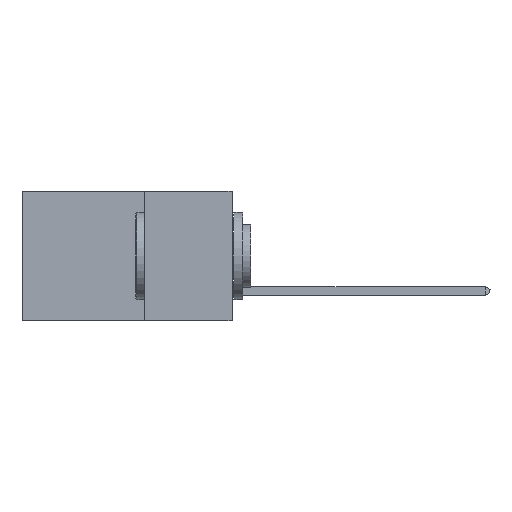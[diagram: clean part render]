
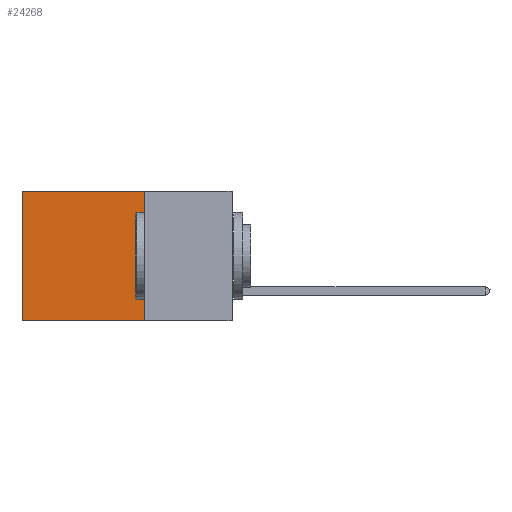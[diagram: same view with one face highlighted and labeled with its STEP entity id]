
A CAD part, left-side view. The second image highlights one B-rep face of the part: STEP entity #24268.
In plain terms, the highlighted planar face has unit normal (-1, 0, 0).
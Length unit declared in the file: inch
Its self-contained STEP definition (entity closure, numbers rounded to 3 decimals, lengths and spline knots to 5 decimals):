
#7 = ORIENTED_EDGE ( 'NONE', *, *, #32468, .F. ) ;
#104 = LINE ( 'NONE', #16611, #7151 ) ;
#862 = VERTEX_POINT ( 'NONE', #12996 ) ;
#2606 = LINE ( 'NONE', #25708, #44000 ) ;
#4894 = EDGE_CURVE ( 'NONE', #24245, #862, #31543, .T. ) ;
#5495 = CARTESIAN_POINT ( 'NONE',  ( 0.2875, 0.25, 0. ) ) ;
#5816 = CARTESIAN_POINT ( 'NONE',  ( 0.2875, 0.25, 0. ) ) ;
#6486 = VECTOR ( 'NONE', #27699, 39.37008 ) ;
#6869 = ORIENTED_EDGE ( 'NONE', *, *, #26207, .T. ) ;
#7151 = VECTOR ( 'NONE', #40931, 39.37008 ) ;
#7490 = CARTESIAN_POINT ( 'NONE',  ( 0.2875, 0.25, -0.37 ) ) ;
#8475 = DIRECTION ( 'NONE',  ( 0., 0., -1. ) ) ;
#10782 = VECTOR ( 'NONE', #38399, 39.37008 ) ;
#11409 = VERTEX_POINT ( 'NONE', #7490 ) ;
#12547 = DIRECTION ( 'NONE',  ( 0., 0., -1. ) ) ;
#12996 = CARTESIAN_POINT ( 'NONE',  ( 0.2875, 0.6, 0. ) ) ;
#16611 = CARTESIAN_POINT ( 'NONE',  ( 0.2875, 0.25, -0.37 ) ) ;
#19975 = EDGE_LOOP ( 'NONE', ( #6869, #7, #23377, #36770 ) ) ;
#21014 = EDGE_CURVE ( 'NONE', #24245, #11409, #2606, .T. ) ;
#23377 = ORIENTED_EDGE ( 'NONE', *, *, #21014, .F. ) ;
#24245 = VERTEX_POINT ( 'NONE', #5816 ) ;
#24268 = ADVANCED_FACE ( 'NONE', ( #33930 ), #37064, .F. ) ;
#25708 = CARTESIAN_POINT ( 'NONE',  ( 0.2875, 0.25, 0. ) ) ;
#26207 = EDGE_CURVE ( 'NONE', #862, #26811, #30447, .T. ) ;
#26811 = VERTEX_POINT ( 'NONE', #32030 ) ;
#27699 = DIRECTION ( 'NONE',  ( 0., 1., 0. ) ) ;
#30447 = LINE ( 'NONE', #38998, #10782 ) ;
#31235 = AXIS2_PLACEMENT_3D ( 'NONE', #5495, #37395, #12547 ) ;
#31543 = LINE ( 'NONE', #33187, #6486 ) ;
#32030 = CARTESIAN_POINT ( 'NONE',  ( 0.2875, 0.6, -0.37 ) ) ;
#32468 = EDGE_CURVE ( 'NONE', #11409, #26811, #104, .T. ) ;
#33187 = CARTESIAN_POINT ( 'NONE',  ( 0.2875, 0.25, 0. ) ) ;
#33930 = FACE_OUTER_BOUND ( 'NONE', #19975, .T. ) ;
#36770 = ORIENTED_EDGE ( 'NONE', *, *, #4894, .T. ) ;
#37064 = PLANE ( 'NONE',  #31235 ) ;
#37395 = DIRECTION ( 'NONE',  ( 1., 0., 0. ) ) ;
#38399 = DIRECTION ( 'NONE',  ( 0., 0., -1. ) ) ;
#38998 = CARTESIAN_POINT ( 'NONE',  ( 0.2875, 0.6, 0. ) ) ;
#40931 = DIRECTION ( 'NONE',  ( 0., 1., 0. ) ) ;
#44000 = VECTOR ( 'NONE', #8475, 39.37008 ) ;
